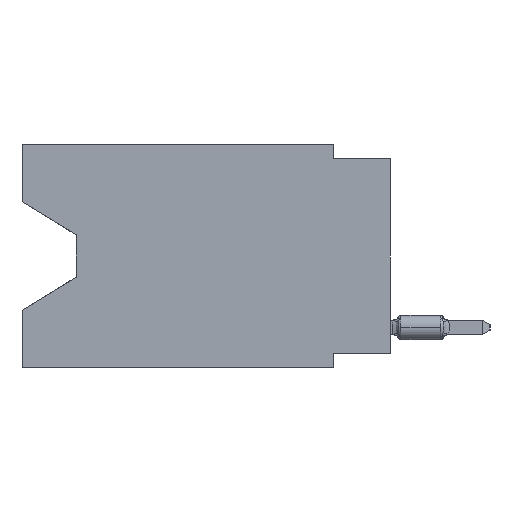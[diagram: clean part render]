
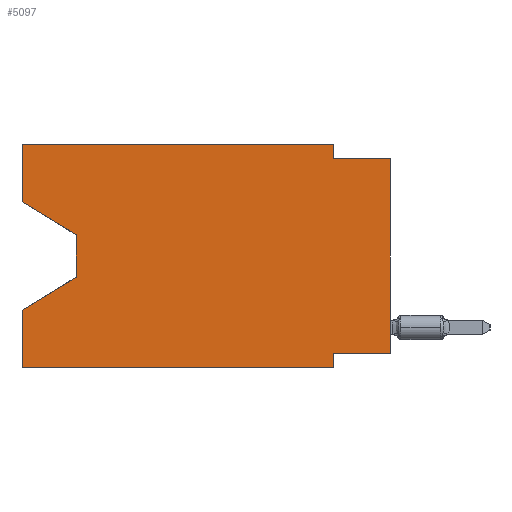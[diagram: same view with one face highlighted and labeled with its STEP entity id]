
A CAD part, left-side view. The second image highlights one B-rep face of the part: STEP entity #5097.
In plain terms, the highlighted planar face has unit normal (-1, 0, 0).
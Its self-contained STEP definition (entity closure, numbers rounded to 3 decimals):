
#79 = LINE ( 'NONE', #38884, #13434 ) ;
#649 = VECTOR ( 'NONE', #24711, 1000. ) ;
#1459 = CARTESIAN_POINT ( 'NONE',  ( 0., 2.54, -9.906 ) ) ;
#1491 = DIRECTION ( 'NONE',  ( 0., 0., 1. ) ) ;
#1493 = VERTEX_POINT ( 'NONE', #35831 ) ;
#1680 = ORIENTED_EDGE ( 'NONE', *, *, #44074, .F. ) ;
#2137 = CARTESIAN_POINT ( 'NONE',  ( 0., 2.54, 0. ) ) ;
#4036 = VERTEX_POINT ( 'NONE', #14029 ) ;
#4616 = CARTESIAN_POINT ( 'NONE',  ( 0., 2.54, 0. ) ) ;
#4726 = CARTESIAN_POINT ( 'NONE',  ( 0., 0., -9.271 ) ) ;
#4971 = VERTEX_POINT ( 'NONE', #17709 ) ;
#5097 = ADVANCED_FACE ( 'NONE', ( #15096 ), #39825, .F. ) ;
#5911 = EDGE_CURVE ( 'NONE', #13647, #1493, #19543, .T. ) ;
#6622 = CARTESIAN_POINT ( 'NONE',  ( 0., 16.383, -2.546 ) ) ;
#6793 = ORIENTED_EDGE ( 'NONE', *, *, #21096, .T. ) ;
#7395 = ORIENTED_EDGE ( 'NONE', *, *, #31401, .F. ) ;
#7952 = DIRECTION ( 'NONE',  ( 1., 0., 0. ) ) ;
#8296 = DIRECTION ( 'NONE',  ( 0., 0.855, -0.519 ) ) ;
#8342 = DIRECTION ( 'NONE',  ( 0., -1., 0. ) ) ;
#8624 = CARTESIAN_POINT ( 'NONE',  ( 0., 16.383, 0. ) ) ;
#8659 = CARTESIAN_POINT ( 'NONE',  ( 0., 13.97, -5.893 ) ) ;
#10062 = CARTESIAN_POINT ( 'NONE',  ( 0., 16.383, 0. ) ) ;
#10550 = CARTESIAN_POINT ( 'NONE',  ( 0., 2.54, -9.271 ) ) ;
#10571 = ORIENTED_EDGE ( 'NONE', *, *, #36212, .T. ) ;
#11496 = LINE ( 'NONE', #15082, #15686 ) ;
#12314 = ORIENTED_EDGE ( 'NONE', *, *, #42318, .T. ) ;
#12607 = EDGE_LOOP ( 'NONE', ( #45942, #10571, #6793, #34111, #12314, #46031, #33113, #18325, #1680, #7395, #16206, #46904 ) ) ;
#12844 = VERTEX_POINT ( 'NONE', #19033 ) ;
#13434 = VECTOR ( 'NONE', #24606, 1000. ) ;
#13647 = VERTEX_POINT ( 'NONE', #10550 ) ;
#14029 = CARTESIAN_POINT ( 'NONE',  ( 0., 16.383, -9.906 ) ) ;
#15082 = CARTESIAN_POINT ( 'NONE',  ( 0., 13.97, -4.013 ) ) ;
#15096 = FACE_OUTER_BOUND ( 'NONE', #12607, .T. ) ;
#15121 = CARTESIAN_POINT ( 'NONE',  ( 0., 0., -0.635 ) ) ;
#15686 = VECTOR ( 'NONE', #44342, 1000. ) ;
#16177 = EDGE_CURVE ( 'NONE', #29045, #13647, #33515, .T. ) ;
#16206 = ORIENTED_EDGE ( 'NONE', *, *, #40272, .F. ) ;
#16356 = CARTESIAN_POINT ( 'NONE',  ( 0., 13.97, -5.893 ) ) ;
#16652 = LINE ( 'NONE', #40931, #45299 ) ;
#17338 = LINE ( 'NONE', #6622, #649 ) ;
#17429 = VERTEX_POINT ( 'NONE', #15121 ) ;
#17709 = CARTESIAN_POINT ( 'NONE',  ( 0., 16.383, -2.546 ) ) ;
#17849 = VERTEX_POINT ( 'NONE', #44576 ) ;
#18325 = ORIENTED_EDGE ( 'NONE', *, *, #21700, .T. ) ;
#18841 = DIRECTION ( 'NONE',  ( 0., 0., -1. ) ) ;
#19033 = CARTESIAN_POINT ( 'NONE',  ( 0., 16.383, 0. ) ) ;
#19543 = LINE ( 'NONE', #1459, #40453 ) ;
#19975 = LINE ( 'NONE', #2137, #22477 ) ;
#21096 = EDGE_CURVE ( 'NONE', #35686, #38557, #44940, .T. ) ;
#21700 = EDGE_CURVE ( 'NONE', #29045, #17429, #46501, .T. ) ;
#22477 = VECTOR ( 'NONE', #41626, 1000. ) ;
#24599 = DIRECTION ( 'NONE',  ( 0., -1., 0. ) ) ;
#24606 = DIRECTION ( 'NONE',  ( 0., 0., 1. ) ) ;
#24711 = DIRECTION ( 'NONE',  ( 0., -0.855, -0.519 ) ) ;
#24815 = VECTOR ( 'NONE', #35355, 1000. ) ;
#28072 = VECTOR ( 'NONE', #41608, 1000. ) ;
#28973 = AXIS2_PLACEMENT_3D ( 'NONE', #29611, #7952, #33406 ) ;
#29045 = VERTEX_POINT ( 'NONE', #36494 ) ;
#29611 = CARTESIAN_POINT ( 'NONE',  ( 0., 16.383, 0. ) ) ;
#31401 = EDGE_CURVE ( 'NONE', #33449, #17849, #19975, .T. ) ;
#32881 = LINE ( 'NONE', #10062, #38330 ) ;
#33113 = ORIENTED_EDGE ( 'NONE', *, *, #16177, .F. ) ;
#33406 = DIRECTION ( 'NONE',  ( 0., 0., -1. ) ) ;
#33449 = VERTEX_POINT ( 'NONE', #4616 ) ;
#33515 = LINE ( 'NONE', #4726, #28072 ) ;
#33986 = EDGE_CURVE ( 'NONE', #4971, #41179, #17338, .T. ) ;
#34111 = ORIENTED_EDGE ( 'NONE', *, *, #36633, .F. ) ;
#35129 = LINE ( 'NONE', #45882, #24815 ) ;
#35355 = DIRECTION ( 'NONE',  ( 0., -1., 0. ) ) ;
#35686 = VERTEX_POINT ( 'NONE', #8659 ) ;
#35831 = CARTESIAN_POINT ( 'NONE',  ( 0., 2.54, -9.906 ) ) ;
#36212 = EDGE_CURVE ( 'NONE', #41179, #35686, #11496, .T. ) ;
#36224 = DIRECTION ( 'NONE',  ( 0., 0., 1. ) ) ;
#36463 = CARTESIAN_POINT ( 'NONE',  ( 0., 0., 0. ) ) ;
#36494 = CARTESIAN_POINT ( 'NONE',  ( 0., 0., -9.271 ) ) ;
#36633 = EDGE_CURVE ( 'NONE', #4036, #38557, #79, .T. ) ;
#38330 = VECTOR ( 'NONE', #24599, 1000. ) ;
#38557 = VERTEX_POINT ( 'NONE', #41567 ) ;
#38624 = VECTOR ( 'NONE', #36224, 1000. ) ;
#38884 = CARTESIAN_POINT ( 'NONE',  ( 0., 16.383, 0. ) ) ;
#39290 = VECTOR ( 'NONE', #8296, 1000. ) ;
#39825 = PLANE ( 'NONE',  #28973 ) ;
#40272 = EDGE_CURVE ( 'NONE', #12844, #33449, #32881, .T. ) ;
#40453 = VECTOR ( 'NONE', #18841, 1000. ) ;
#40498 = LINE ( 'NONE', #8624, #42508 ) ;
#40931 = CARTESIAN_POINT ( 'NONE',  ( 0., 16.383, -9.906 ) ) ;
#41179 = VERTEX_POINT ( 'NONE', #41742 ) ;
#41429 = EDGE_CURVE ( 'NONE', #4971, #12844, #40498, .T. ) ;
#41567 = CARTESIAN_POINT ( 'NONE',  ( 0., 16.383, -7.36 ) ) ;
#41608 = DIRECTION ( 'NONE',  ( 0., 1., 0. ) ) ;
#41626 = DIRECTION ( 'NONE',  ( 0., 0., -1. ) ) ;
#41742 = CARTESIAN_POINT ( 'NONE',  ( 0., 13.97, -4.013 ) ) ;
#42318 = EDGE_CURVE ( 'NONE', #4036, #1493, #16652, .T. ) ;
#42508 = VECTOR ( 'NONE', #1491, 1000. ) ;
#44074 = EDGE_CURVE ( 'NONE', #17849, #17429, #35129, .T. ) ;
#44342 = DIRECTION ( 'NONE',  ( 0., 0., -1. ) ) ;
#44576 = CARTESIAN_POINT ( 'NONE',  ( 0., 2.54, -0.635 ) ) ;
#44940 = LINE ( 'NONE', #16356, #39290 ) ;
#45299 = VECTOR ( 'NONE', #8342, 1000. ) ;
#45882 = CARTESIAN_POINT ( 'NONE',  ( 0., 0., -0.635 ) ) ;
#45942 = ORIENTED_EDGE ( 'NONE', *, *, #33986, .T. ) ;
#46031 = ORIENTED_EDGE ( 'NONE', *, *, #5911, .F. ) ;
#46501 = LINE ( 'NONE', #36463, #38624 ) ;
#46904 = ORIENTED_EDGE ( 'NONE', *, *, #41429, .F. ) ;
